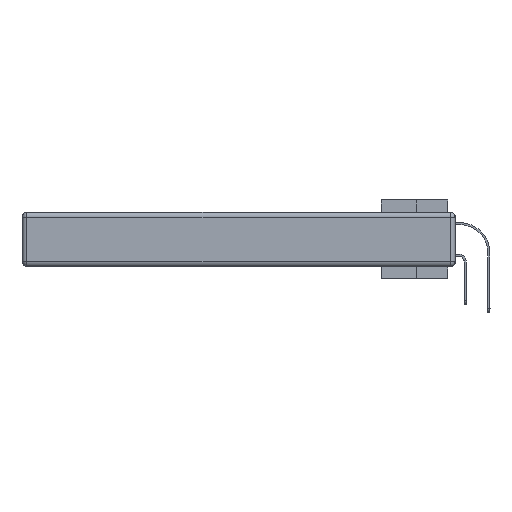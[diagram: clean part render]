
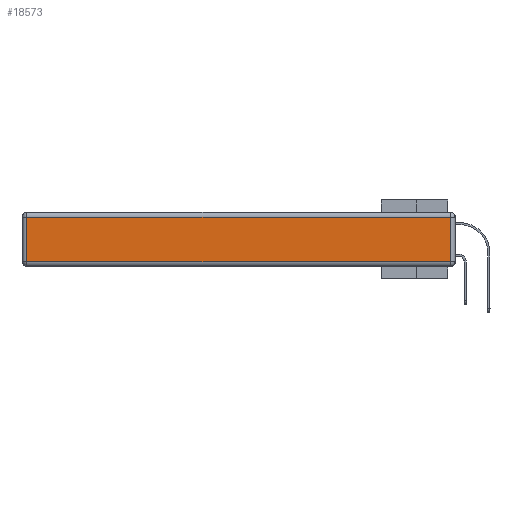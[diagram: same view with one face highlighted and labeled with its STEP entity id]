
A CAD part, left-side view. The second image highlights one B-rep face of the part: STEP entity #18573.
In plain terms, the highlighted planar face has unit normal (-1, 0, 0).
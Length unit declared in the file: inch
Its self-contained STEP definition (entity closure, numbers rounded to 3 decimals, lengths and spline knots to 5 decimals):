
#86 = LINE ( 'NONE', #19469, #2488 ) ;
#179 = CARTESIAN_POINT ( 'NONE',  ( 0., 0.03, -0.343 ) ) ;
#2488 = VECTOR ( 'NONE', #16947, 39.37008 ) ;
#3091 = CARTESIAN_POINT ( 'NONE',  ( 0., 2.72, -0.03 ) ) ;
#4828 = CARTESIAN_POINT ( 'NONE',  ( 0., 2.72, -0.343 ) ) ;
#8686 = DIRECTION ( 'NONE',  ( -1., 0., 0. ) ) ;
#8800 = LINE ( 'NONE', #179, #34201 ) ;
#10077 = DIRECTION ( 'NONE',  ( 0., 1., 0. ) ) ;
#10564 = VERTEX_POINT ( 'NONE', #29500 ) ;
#11026 = PLANE ( 'NONE',  #25455 ) ;
#12700 = ORIENTED_EDGE ( 'NONE', *, *, #33446, .T. ) ;
#12800 = EDGE_CURVE ( 'NONE', #30880, #27197, #29942, .T. ) ;
#12847 = CARTESIAN_POINT ( 'NONE',  ( 0., 0.03, -0.313 ) ) ;
#14612 = VECTOR ( 'NONE', #10077, 39.37008 ) ;
#15585 = ORIENTED_EDGE ( 'NONE', *, *, #23439, .T. ) ;
#16130 = DIRECTION ( 'NONE',  ( 0., 0., -1. ) ) ;
#16947 = DIRECTION ( 'NONE',  ( 0., -1., 0. ) ) ;
#18573 = ADVANCED_FACE ( 'NONE', ( #25185 ), #11026, .T. ) ;
#19469 = CARTESIAN_POINT ( 'NONE',  ( 0., 0., -0.313 ) ) ;
#19617 = DIRECTION ( 'NONE',  ( 0., 0., 1. ) ) ;
#20243 = ORIENTED_EDGE ( 'NONE', *, *, #12800, .T. ) ;
#21918 = VERTEX_POINT ( 'NONE', #12847 ) ;
#23439 = EDGE_CURVE ( 'NONE', #27197, #21918, #86, .T. ) ;
#25185 = FACE_OUTER_BOUND ( 'NONE', #32694, .T. ) ;
#25350 = VECTOR ( 'NONE', #16130, 39.37008 ) ;
#25455 = AXIS2_PLACEMENT_3D ( 'NONE', #29859, #8686, #19617 ) ;
#27197 = VERTEX_POINT ( 'NONE', #32133 ) ;
#27356 = EDGE_CURVE ( 'NONE', #21918, #10564, #8800, .T. ) ;
#29094 = LINE ( 'NONE', #29622, #14612 ) ;
#29500 = CARTESIAN_POINT ( 'NONE',  ( 0., 0.03, -0.03 ) ) ;
#29622 = CARTESIAN_POINT ( 'NONE',  ( 0., 2.75, -0.03 ) ) ;
#29859 = CARTESIAN_POINT ( 'NONE',  ( 0., 0., -0.343 ) ) ;
#29942 = LINE ( 'NONE', #4828, #25350 ) ;
#30511 = DIRECTION ( 'NONE',  ( 0., 0., 1. ) ) ;
#30880 = VERTEX_POINT ( 'NONE', #3091 ) ;
#31908 = ORIENTED_EDGE ( 'NONE', *, *, #27356, .T. ) ;
#32133 = CARTESIAN_POINT ( 'NONE',  ( 0., 2.72, -0.313 ) ) ;
#32694 = EDGE_LOOP ( 'NONE', ( #15585, #31908, #12700, #20243 ) ) ;
#33446 = EDGE_CURVE ( 'NONE', #10564, #30880, #29094, .T. ) ;
#34201 = VECTOR ( 'NONE', #30511, 39.37008 ) ;
